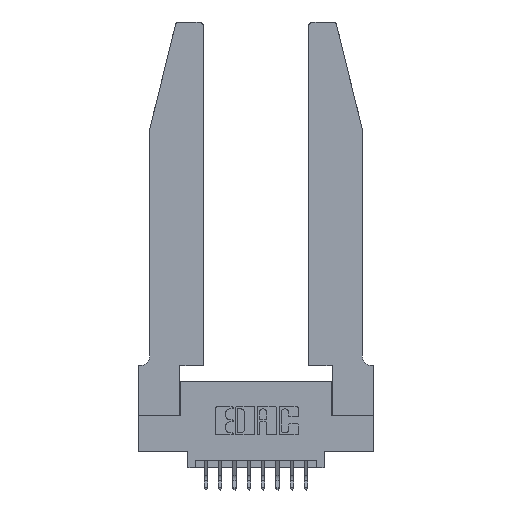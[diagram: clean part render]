
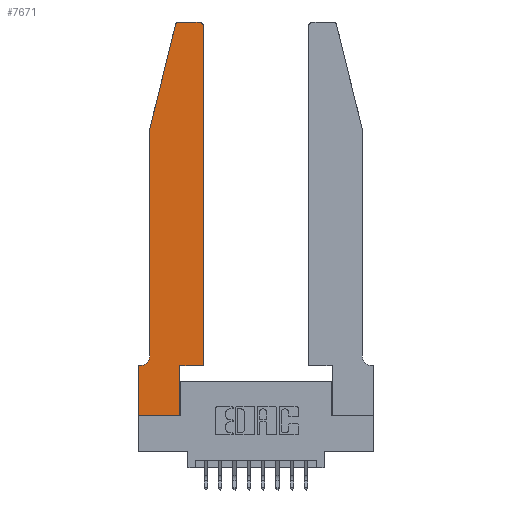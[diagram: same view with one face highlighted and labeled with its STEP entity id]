
A CAD part, top view. The second image highlights one B-rep face of the part: STEP entity #7671.
In plain terms, the highlighted planar face has unit normal (0, 0, 1).
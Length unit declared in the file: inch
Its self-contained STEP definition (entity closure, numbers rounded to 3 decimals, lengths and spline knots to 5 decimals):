
#135 = LINE ( 'NONE', #14677, #6924 ) ;
#242 = LINE ( 'NONE', #11246, #3673 ) ;
#305 = ORIENTED_EDGE ( 'NONE', *, *, #1140, .T. ) ;
#540 = PLANE ( 'NONE',  #13288 ) ;
#756 = VERTEX_POINT ( 'NONE', #7018 ) ;
#791 = DIRECTION ( 'NONE',  ( 0., 0., 1. ) ) ;
#816 = VECTOR ( 'NONE', #11228, 39.37008 ) ;
#850 = EDGE_CURVE ( 'NONE', #3844, #1339, #4196, .T. ) ;
#876 = VECTOR ( 'NONE', #2633, 39.37008 ) ;
#1003 = LINE ( 'NONE', #6153, #3983 ) ;
#1105 = ORIENTED_EDGE ( 'NONE', *, *, #14045, .T. ) ;
#1140 = EDGE_CURVE ( 'NONE', #1339, #6223, #3214, .T. ) ;
#1339 = VERTEX_POINT ( 'NONE', #10441 ) ;
#1650 = CARTESIAN_POINT ( 'NONE',  ( 0.0755, 0.35, 0.37 ) ) ;
#1866 = DIRECTION ( 'NONE',  ( 0., 0., 1. ) ) ;
#2223 = VERTEX_POINT ( 'NONE', #15605 ) ;
#2406 = FACE_OUTER_BOUND ( 'NONE', #2879, .T. ) ;
#2633 = DIRECTION ( 'NONE',  ( 0., -1., 0. ) ) ;
#2721 = ORIENTED_EDGE ( 'NONE', *, *, #6174, .T. ) ;
#2879 = EDGE_LOOP ( 'NONE', ( #10964, #10251, #2721, #13458, #305, #1105, #10749, #14078, #7945, #6312, #10033, #12686 ) ) ;
#3214 = CIRCLE ( 'NONE', #5892, 0.07 ) ;
#3415 = CARTESIAN_POINT ( 'NONE',  ( 0.4505, 0.35, 0.37 ) ) ;
#3670 = CARTESIAN_POINT ( 'NONE',  ( 0.4505, 0.35, 0.37 ) ) ;
#3673 = VECTOR ( 'NONE', #3883, 39.37008 ) ;
#3844 = VERTEX_POINT ( 'NONE', #10689 ) ;
#3883 = DIRECTION ( 'NONE',  ( 1., 0., 0. ) ) ;
#3983 = VECTOR ( 'NONE', #12220, 39.37008 ) ;
#4104 = VERTEX_POINT ( 'NONE', #5060 ) ;
#4196 = LINE ( 'NONE', #11834, #816 ) ;
#4284 = CARTESIAN_POINT ( 'NONE',  ( 0.4205, 2.75, 0.37 ) ) ;
#4530 = CARTESIAN_POINT ( 'NONE',  ( 0.2865, 0.35, 0.37 ) ) ;
#4674 = DIRECTION ( 'NONE',  ( 1., 0., 0. ) ) ;
#4921 = CARTESIAN_POINT ( 'NONE',  ( 0., 0.35, 0.37 ) ) ;
#5060 = CARTESIAN_POINT ( 'NONE',  ( 0.2865, 0., 0.37 ) ) ;
#5802 = VECTOR ( 'NONE', #4674, 39.37008 ) ;
#5892 = AXIS2_PLACEMENT_3D ( 'NONE', #15942, #11096, #11042 ) ;
#6153 = CARTESIAN_POINT ( 'NONE',  ( 0.2865, 0.35, 0.37 ) ) ;
#6174 = EDGE_CURVE ( 'NONE', #9383, #3844, #13802, .T. ) ;
#6199 = EDGE_CURVE ( 'NONE', #7189, #4104, #242, .T. ) ;
#6223 = VERTEX_POINT ( 'NONE', #8894 ) ;
#6312 = ORIENTED_EDGE ( 'NONE', *, *, #11514, .T. ) ;
#6664 = VERTEX_POINT ( 'NONE', #4921 ) ;
#6854 = CARTESIAN_POINT ( 'NONE',  ( 0.4205, 2.72, 0.37 ) ) ;
#6924 = VECTOR ( 'NONE', #7486, 39.37008 ) ;
#7018 = CARTESIAN_POINT ( 'NONE',  ( 0.4505, 2.72, 0.37 ) ) ;
#7189 = VERTEX_POINT ( 'NONE', #8531 ) ;
#7486 = DIRECTION ( 'NONE',  ( -1., 0., 0. ) ) ;
#7671 = ADVANCED_FACE ( 'NONE', ( #2406 ), #540, .T. ) ;
#7945 = ORIENTED_EDGE ( 'NONE', *, *, #14424, .T. ) ;
#8083 = DIRECTION ( 'NONE',  ( 1., 0., 0. ) ) ;
#8176 = CARTESIAN_POINT ( 'NONE',  ( 0.25487, 2.72718, 0.37 ) ) ;
#8332 = CARTESIAN_POINT ( 'NONE',  ( 0.284, 2.72, 0.37 ) ) ;
#8526 = CIRCLE ( 'NONE', #15821, 0.03 ) ;
#8531 = CARTESIAN_POINT ( 'NONE',  ( 0., 0., 0.37 ) ) ;
#8796 = CARTESIAN_POINT ( 'NONE',  ( 0.0755, 2., 0.37 ) ) ;
#8894 = CARTESIAN_POINT ( 'NONE',  ( 0.0055, 0.35, 0.37 ) ) ;
#9051 = VECTOR ( 'NONE', #12748, 39.37008 ) ;
#9122 = VECTOR ( 'NONE', #11046, 39.37008 ) ;
#9319 = CARTESIAN_POINT ( 'NONE',  ( 0., 0.35, 0.37 ) ) ;
#9383 = VERTEX_POINT ( 'NONE', #8176 ) ;
#9442 = EDGE_CURVE ( 'NONE', #2223, #9383, #14558, .T. ) ;
#9554 = DIRECTION ( 'NONE',  ( 1., 0., 0. ) ) ;
#10033 = ORIENTED_EDGE ( 'NONE', *, *, #10117, .T. ) ;
#10047 = CARTESIAN_POINT ( 'NONE',  ( 0., 0., 0.37 ) ) ;
#10117 = EDGE_CURVE ( 'NONE', #11720, #756, #15085, .T. ) ;
#10195 = EDGE_CURVE ( 'NONE', #6664, #7189, #13629, .T. ) ;
#10251 = ORIENTED_EDGE ( 'NONE', *, *, #9442, .T. ) ;
#10441 = CARTESIAN_POINT ( 'NONE',  ( 0.0755, 0.42, 0.37 ) ) ;
#10517 = DIRECTION ( 'NONE',  ( 1., 0., 0. ) ) ;
#10689 = CARTESIAN_POINT ( 'NONE',  ( 0.0755, 2., 0.37 ) ) ;
#10749 = ORIENTED_EDGE ( 'NONE', *, *, #10195, .T. ) ;
#10839 = EDGE_CURVE ( 'NONE', #756, #15796, #8526, .T. ) ;
#10964 = ORIENTED_EDGE ( 'NONE', *, *, #14936, .T. ) ;
#10991 = VECTOR ( 'NONE', #15943, 39.37008 ) ;
#10992 = VERTEX_POINT ( 'NONE', #4530 ) ;
#11042 = DIRECTION ( 'NONE',  ( -1., 0., 0. ) ) ;
#11046 = DIRECTION ( 'NONE',  ( 0., 1., 0. ) ) ;
#11096 = DIRECTION ( 'NONE',  ( 0., 0., -1. ) ) ;
#11228 = DIRECTION ( 'NONE',  ( 0., -1., 0. ) ) ;
#11246 = CARTESIAN_POINT ( 'NONE',  ( 0., 0., 0.37 ) ) ;
#11514 = EDGE_CURVE ( 'NONE', #10992, #11720, #11893, .T. ) ;
#11720 = VERTEX_POINT ( 'NONE', #12440 ) ;
#11834 = CARTESIAN_POINT ( 'NONE',  ( 0.0755, 2., 0.37 ) ) ;
#11893 = LINE ( 'NONE', #3415, #5802 ) ;
#12220 = DIRECTION ( 'NONE',  ( 0., 1., 0. ) ) ;
#12264 = LINE ( 'NONE', #1650, #9051 ) ;
#12440 = CARTESIAN_POINT ( 'NONE',  ( 0.4505, 0.35, 0.37 ) ) ;
#12602 = AXIS2_PLACEMENT_3D ( 'NONE', #8332, #791, #9554 ) ;
#12686 = ORIENTED_EDGE ( 'NONE', *, *, #10839, .T. ) ;
#12748 = DIRECTION ( 'NONE',  ( -1., 0., 0. ) ) ;
#13288 = AXIS2_PLACEMENT_3D ( 'NONE', #9319, #1866, #10517 ) ;
#13458 = ORIENTED_EDGE ( 'NONE', *, *, #850, .T. ) ;
#13629 = LINE ( 'NONE', #10047, #876 ) ;
#13802 = LINE ( 'NONE', #8796, #10991 ) ;
#14045 = EDGE_CURVE ( 'NONE', #6223, #6664, #12264, .T. ) ;
#14078 = ORIENTED_EDGE ( 'NONE', *, *, #6199, .T. ) ;
#14424 = EDGE_CURVE ( 'NONE', #4104, #10992, #1003, .T. ) ;
#14558 = CIRCLE ( 'NONE', #12602, 0.03 ) ;
#14677 = CARTESIAN_POINT ( 'NONE',  ( 0.2605, 2.75, 0.37 ) ) ;
#14936 = EDGE_CURVE ( 'NONE', #15796, #2223, #135, .T. ) ;
#15085 = LINE ( 'NONE', #3670, #9122 ) ;
#15242 = DIRECTION ( 'NONE',  ( 0., 0., 1. ) ) ;
#15605 = CARTESIAN_POINT ( 'NONE',  ( 0.284, 2.75, 0.37 ) ) ;
#15796 = VERTEX_POINT ( 'NONE', #4284 ) ;
#15821 = AXIS2_PLACEMENT_3D ( 'NONE', #6854, #15242, #8083 ) ;
#15942 = CARTESIAN_POINT ( 'NONE',  ( 0.0055, 0.42, 0.37 ) ) ;
#15943 = DIRECTION ( 'NONE',  ( -0.239, -0.971, 0. ) ) ;
